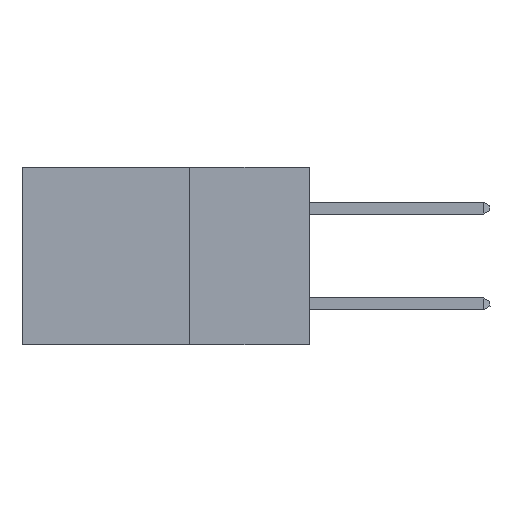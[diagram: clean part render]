
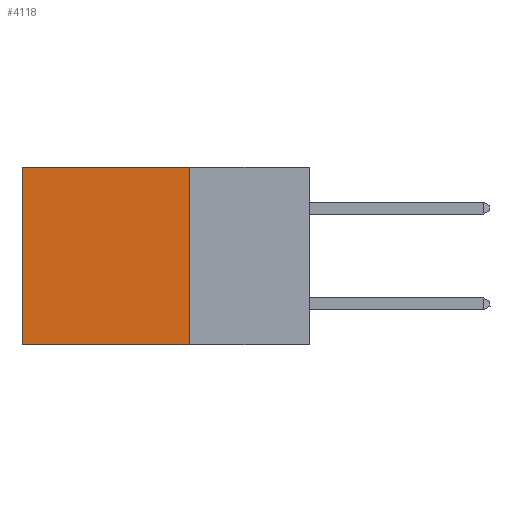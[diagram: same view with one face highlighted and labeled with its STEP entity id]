
A CAD part, left-side view. The second image highlights one B-rep face of the part: STEP entity #4118.
In plain terms, the highlighted planar face has unit normal (-1, 0, 0).
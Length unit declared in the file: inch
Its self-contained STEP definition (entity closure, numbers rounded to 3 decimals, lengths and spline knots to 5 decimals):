
#933 = FACE_OUTER_BOUND ( 'NONE', #3630, .T. ) ;
#1032 = CARTESIAN_POINT ( 'NONE',  ( 0.2875, 0.25, -0.37 ) ) ;
#1344 = CARTESIAN_POINT ( 'NONE',  ( 0.2875, 0.25, 0. ) ) ;
#1524 = ORIENTED_EDGE ( 'NONE', *, *, #3807, .F. ) ;
#2014 = VECTOR ( 'NONE', #7501, 39.37008 ) ;
#3630 = EDGE_LOOP ( 'NONE', ( #6669, #1524, #12339, #13659 ) ) ;
#3800 = CARTESIAN_POINT ( 'NONE',  ( 0.2875, 0.25, 0. ) ) ;
#3807 = EDGE_CURVE ( 'NONE', #14146, #11570, #11838, .T. ) ;
#4118 = ADVANCED_FACE ( 'NONE', ( #933 ), #13789, .F. ) ;
#4334 = VECTOR ( 'NONE', #4687, 39.37008 ) ;
#4687 = DIRECTION ( 'NONE',  ( 0., 0., -1. ) ) ;
#4699 = LINE ( 'NONE', #11715, #4334 ) ;
#4755 = VECTOR ( 'NONE', #7552, 39.37008 ) ;
#5288 = LINE ( 'NONE', #14241, #4755 ) ;
#6669 = ORIENTED_EDGE ( 'NONE', *, *, #11190, .T. ) ;
#6709 = CARTESIAN_POINT ( 'NONE',  ( 0.2875, 0.6, 0. ) ) ;
#7501 = DIRECTION ( 'NONE',  ( 0., 1., 0. ) ) ;
#7552 = DIRECTION ( 'NONE',  ( 0., 1., 0. ) ) ;
#8453 = CARTESIAN_POINT ( 'NONE',  ( 0.2875, 0.6, 0. ) ) ;
#9077 = DIRECTION ( 'NONE',  ( 0., 0., -1. ) ) ;
#10032 = VERTEX_POINT ( 'NONE', #3800 ) ;
#10164 = LINE ( 'NONE', #6709, #13528 ) ;
#10439 = DIRECTION ( 'NONE',  ( 1., 0., 0. ) ) ;
#10485 = VERTEX_POINT ( 'NONE', #8453 ) ;
#10495 = DIRECTION ( 'NONE',  ( 0., 0., -1. ) ) ;
#10714 = CARTESIAN_POINT ( 'NONE',  ( 0.2875, 0.6, -0.37 ) ) ;
#11022 = AXIS2_PLACEMENT_3D ( 'NONE', #1344, #10439, #10495 ) ;
#11026 = CARTESIAN_POINT ( 'NONE',  ( 0.2875, 0.25, -0.37 ) ) ;
#11190 = EDGE_CURVE ( 'NONE', #10485, #11570, #10164, .T. ) ;
#11570 = VERTEX_POINT ( 'NONE', #10714 ) ;
#11715 = CARTESIAN_POINT ( 'NONE',  ( 0.2875, 0.25, 0. ) ) ;
#11838 = LINE ( 'NONE', #11026, #2014 ) ;
#12197 = EDGE_CURVE ( 'NONE', #10032, #10485, #5288, .T. ) ;
#12339 = ORIENTED_EDGE ( 'NONE', *, *, #14358, .F. ) ;
#13528 = VECTOR ( 'NONE', #9077, 39.37008 ) ;
#13659 = ORIENTED_EDGE ( 'NONE', *, *, #12197, .T. ) ;
#13789 = PLANE ( 'NONE',  #11022 ) ;
#14146 = VERTEX_POINT ( 'NONE', #1032 ) ;
#14241 = CARTESIAN_POINT ( 'NONE',  ( 0.2875, 0.25, 0. ) ) ;
#14358 = EDGE_CURVE ( 'NONE', #10032, #14146, #4699, .T. ) ;
